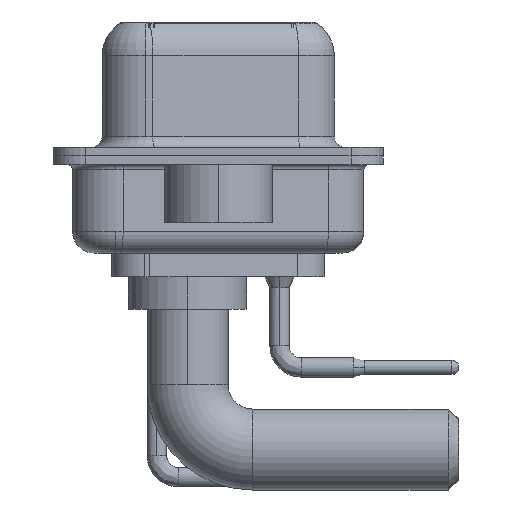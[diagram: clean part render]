
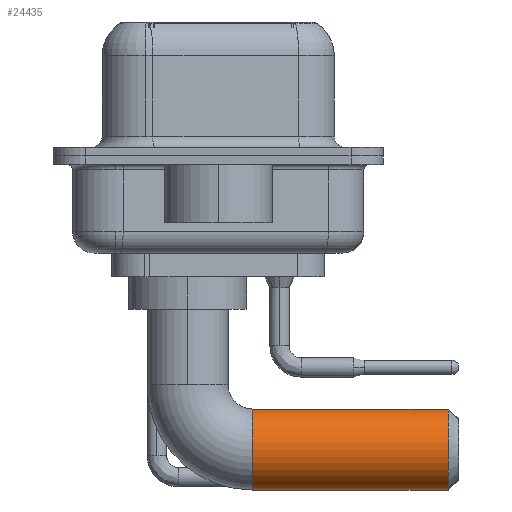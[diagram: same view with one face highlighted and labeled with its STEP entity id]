
A CAD part, left-side view. The second image highlights one B-rep face of the part: STEP entity #24435.
In plain terms, the highlighted cylindrical face has radius 1.875 mm (diameter 3.75 mm), a partial arc.
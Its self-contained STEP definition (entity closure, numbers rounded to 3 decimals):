
#822 = AXIS2_PLACEMENT_3D ( 'NONE', #23462, #7687, #19587 ) ;
#1177 = DIRECTION ( 'NONE',  ( 0., -1., 0. ) ) ;
#1611 = DIRECTION ( 'NONE',  ( -1., 0., 0. ) ) ;
#1621 = VECTOR ( 'NONE', #20850, 1000. ) ;
#1901 = CARTESIAN_POINT ( 'NONE',  ( 0., -12.07, -4.625 ) ) ;
#2216 = CIRCLE ( 'NONE', #26440, 1.875 ) ;
#2450 = EDGE_LOOP ( 'NONE', ( #11680, #8324, #13552, #11926 ) ) ;
#2646 = VERTEX_POINT ( 'NONE', #25578 ) ;
#4169 = EDGE_CURVE ( 'NONE', #18651, #17564, #2216, .T. ) ;
#6169 = CARTESIAN_POINT ( 'NONE',  ( 0., -12.07, -6.5 ) ) ;
#7033 = LINE ( 'NONE', #9403, #1621 ) ;
#7371 = EDGE_CURVE ( 'NONE', #2646, #20002, #15406, .T. ) ;
#7545 = FACE_OUTER_BOUND ( 'NONE', #2450, .T. ) ;
#7687 = DIRECTION ( 'NONE',  ( 0., -1., 0. ) ) ;
#8324 = ORIENTED_EDGE ( 'NONE', *, *, #7371, .T. ) ;
#9403 = CARTESIAN_POINT ( 'NONE',  ( 0., -3., -8.375 ) ) ;
#11680 = ORIENTED_EDGE ( 'NONE', *, *, #24402, .F. ) ;
#11926 = ORIENTED_EDGE ( 'NONE', *, *, #4169, .T. ) ;
#12548 = EDGE_CURVE ( 'NONE', #20002, #18651, #7033, .T. ) ;
#13552 = ORIENTED_EDGE ( 'NONE', *, *, #12548, .T. ) ;
#13646 = CARTESIAN_POINT ( 'NONE',  ( 0., -3., -8.375 ) ) ;
#14989 = CARTESIAN_POINT ( 'NONE',  ( 0., -3., -4.625 ) ) ;
#15406 = CIRCLE ( 'NONE', #19199, 1.875 ) ;
#16606 = CYLINDRICAL_SURFACE ( 'NONE', #822, 1.875 ) ;
#17564 = VERTEX_POINT ( 'NONE', #1901 ) ;
#18027 = CARTESIAN_POINT ( 'NONE',  ( 0., -12.07, -8.375 ) ) ;
#18651 = VERTEX_POINT ( 'NONE', #18027 ) ;
#19199 = AXIS2_PLACEMENT_3D ( 'NONE', #21678, #1177, #1611 ) ;
#19587 = DIRECTION ( 'NONE',  ( 0., 0., -1. ) ) ;
#20002 = VERTEX_POINT ( 'NONE', #13646 ) ;
#20850 = DIRECTION ( 'NONE',  ( 0., -1., 0. ) ) ;
#21678 = CARTESIAN_POINT ( 'NONE',  ( 0., -3., -6.5 ) ) ;
#22058 = DIRECTION ( 'NONE',  ( 0., 1., 0. ) ) ;
#23462 = CARTESIAN_POINT ( 'NONE',  ( 0., -3., -6.5 ) ) ;
#24402 = EDGE_CURVE ( 'NONE', #2646, #17564, #25686, .T. ) ;
#24435 = ADVANCED_FACE ( 'NONE', ( #7545 ), #16606, .T. ) ;
#25578 = CARTESIAN_POINT ( 'NONE',  ( 0., -3., -4.625 ) ) ;
#25686 = LINE ( 'NONE', #14989, #28846 ) ;
#26440 = AXIS2_PLACEMENT_3D ( 'NONE', #6169, #22058, #26525 ) ;
#26525 = DIRECTION ( 'NONE',  ( 0., 0., -1. ) ) ;
#28535 = DIRECTION ( 'NONE',  ( 0., -1., 0. ) ) ;
#28846 = VECTOR ( 'NONE', #28535, 1000. ) ;
